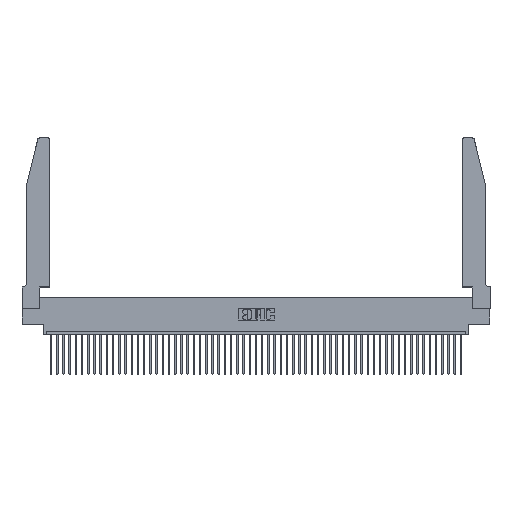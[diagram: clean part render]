
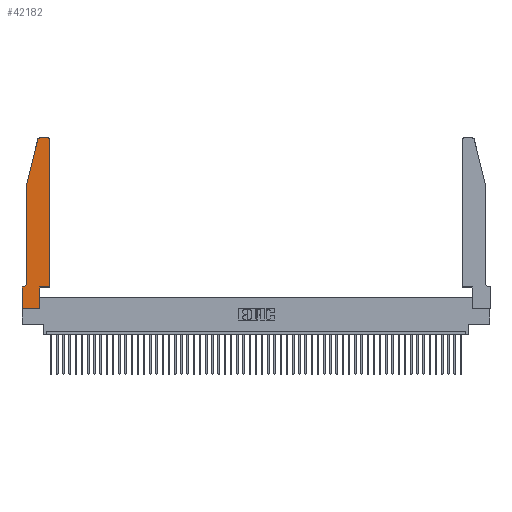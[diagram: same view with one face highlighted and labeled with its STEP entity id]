
A CAD part, top view. The second image highlights one B-rep face of the part: STEP entity #42182.
In plain terms, the highlighted planar face has unit normal (0, 0, 1).
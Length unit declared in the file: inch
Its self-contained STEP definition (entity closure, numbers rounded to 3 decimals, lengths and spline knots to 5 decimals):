
#329 = CARTESIAN_POINT ( 'NONE',  ( 0.0755, 2., 0.37 ) ) ;
#346 = CIRCLE ( 'NONE', #16321, 0.03 ) ;
#608 = CARTESIAN_POINT ( 'NONE',  ( 0.4205, 2.75, 0.37 ) ) ;
#886 = VERTEX_POINT ( 'NONE', #20206 ) ;
#1079 = VERTEX_POINT ( 'NONE', #32939 ) ;
#1158 = CARTESIAN_POINT ( 'NONE',  ( 0.0755, 2., 0.37 ) ) ;
#1181 = CARTESIAN_POINT ( 'NONE',  ( 0.0055, 0.42, 0.37 ) ) ;
#2840 = CARTESIAN_POINT ( 'NONE',  ( 0., 0., 0.37 ) ) ;
#4783 = DIRECTION ( 'NONE',  ( -1., 0., 0. ) ) ;
#4904 = DIRECTION ( 'NONE',  ( 0., 0., 1. ) ) ;
#5257 = DIRECTION ( 'NONE',  ( 0., 0., -1. ) ) ;
#5726 = AXIS2_PLACEMENT_3D ( 'NONE', #1181, #5257, #4783 ) ;
#6434 = EDGE_CURVE ( 'NONE', #24270, #14712, #34978, .T. ) ;
#6566 = VECTOR ( 'NONE', #10923, 39.37008 ) ;
#6941 = CARTESIAN_POINT ( 'NONE',  ( 0.4505, 2.72, 0.37 ) ) ;
#7412 = EDGE_CURVE ( 'NONE', #33512, #45178, #346, .T. ) ;
#9085 = EDGE_CURVE ( 'NONE', #45178, #26135, #44754, .T. ) ;
#9306 = DIRECTION ( 'NONE',  ( -0.239, -0.971, 0. ) ) ;
#10079 = VECTOR ( 'NONE', #38637, 39.37008 ) ;
#10217 = ORIENTED_EDGE ( 'NONE', *, *, #29654, .T. ) ;
#10428 = CARTESIAN_POINT ( 'NONE',  ( 0.4505, 0.35, 0.37 ) ) ;
#10923 = DIRECTION ( 'NONE',  ( 1., 0., 0. ) ) ;
#11467 = DIRECTION ( 'NONE',  ( -1., 0., 0. ) ) ;
#11784 = ORIENTED_EDGE ( 'NONE', *, *, #13520, .T. ) ;
#12671 = CARTESIAN_POINT ( 'NONE',  ( 0.4205, 2.72, 0.37 ) ) ;
#13118 = ORIENTED_EDGE ( 'NONE', *, *, #25463, .T. ) ;
#13520 = EDGE_CURVE ( 'NONE', #48014, #1079, #25300, .T. ) ;
#13732 = ORIENTED_EDGE ( 'NONE', *, *, #50734, .T. ) ;
#13785 = ORIENTED_EDGE ( 'NONE', *, *, #41530, .T. ) ;
#13830 = CARTESIAN_POINT ( 'NONE',  ( 0., 0.35, 0.37 ) ) ;
#14712 = VERTEX_POINT ( 'NONE', #1158 ) ;
#16321 = AXIS2_PLACEMENT_3D ( 'NONE', #12671, #19629, #17444 ) ;
#16602 = CARTESIAN_POINT ( 'NONE',  ( 0.25487, 2.72718, 0.37 ) ) ;
#17444 = DIRECTION ( 'NONE',  ( 1., 0., 0. ) ) ;
#17560 = ORIENTED_EDGE ( 'NONE', *, *, #6434, .T. ) ;
#18526 = ORIENTED_EDGE ( 'NONE', *, *, #9085, .T. ) ;
#19629 = DIRECTION ( 'NONE',  ( 0., 0., 1. ) ) ;
#20206 = CARTESIAN_POINT ( 'NONE',  ( 0.2865, 0., 0.37 ) ) ;
#20846 = LINE ( 'NONE', #45783, #51083 ) ;
#21746 = DIRECTION ( 'NONE',  ( 1., 0., 0. ) ) ;
#21899 = VERTEX_POINT ( 'NONE', #38941 ) ;
#22850 = CARTESIAN_POINT ( 'NONE',  ( 0.2605, 2.75, 0.37 ) ) ;
#23298 = EDGE_CURVE ( 'NONE', #42339, #886, #20846, .T. ) ;
#24270 = VERTEX_POINT ( 'NONE', #16602 ) ;
#24715 = VECTOR ( 'NONE', #26577, 39.37008 ) ;
#24880 = CARTESIAN_POINT ( 'NONE',  ( 0.284, 2.72, 0.37 ) ) ;
#25300 = LINE ( 'NONE', #34911, #6566 ) ;
#25463 = EDGE_CURVE ( 'NONE', #1079, #33512, #35424, .T. ) ;
#26110 = EDGE_CURVE ( 'NONE', #26135, #24270, #37158, .T. ) ;
#26112 = DIRECTION ( 'NONE',  ( 0., 0., 1. ) ) ;
#26135 = VERTEX_POINT ( 'NONE', #30339 ) ;
#26250 = LINE ( 'NONE', #329, #51472 ) ;
#26326 = CARTESIAN_POINT ( 'NONE',  ( 0.2865, 0.35, 0.37 ) ) ;
#26564 = VECTOR ( 'NONE', #38978, 39.37008 ) ;
#26577 = DIRECTION ( 'NONE',  ( 0., 1., 0. ) ) ;
#27135 = ORIENTED_EDGE ( 'NONE', *, *, #26110, .T. ) ;
#27456 = CARTESIAN_POINT ( 'NONE',  ( 0.0755, 2., 0.37 ) ) ;
#27586 = CARTESIAN_POINT ( 'NONE',  ( 0.0755, 0.35, 0.37 ) ) ;
#29398 = CARTESIAN_POINT ( 'NONE',  ( 0.2865, 0.35, 0.37 ) ) ;
#29490 = LINE ( 'NONE', #26326, #10079 ) ;
#29654 = EDGE_CURVE ( 'NONE', #32165, #21899, #34146, .T. ) ;
#29679 = CARTESIAN_POINT ( 'NONE',  ( 0., 0., 0.37 ) ) ;
#29783 = FACE_OUTER_BOUND ( 'NONE', #38321, .T. ) ;
#30339 = CARTESIAN_POINT ( 'NONE',  ( 0.284, 2.75, 0.37 ) ) ;
#30767 = VECTOR ( 'NONE', #41751, 39.37008 ) ;
#32165 = VERTEX_POINT ( 'NONE', #45213 ) ;
#32939 = CARTESIAN_POINT ( 'NONE',  ( 0.4505, 0.35, 0.37 ) ) ;
#33512 = VERTEX_POINT ( 'NONE', #6941 ) ;
#34146 = LINE ( 'NONE', #27586, #50504 ) ;
#34911 = CARTESIAN_POINT ( 'NONE',  ( 0.4505, 0.35, 0.37 ) ) ;
#34978 = LINE ( 'NONE', #27456, #48210 ) ;
#35424 = LINE ( 'NONE', #10428, #24715 ) ;
#35716 = ORIENTED_EDGE ( 'NONE', *, *, #43220, .T. ) ;
#36349 = LINE ( 'NONE', #29679, #30767 ) ;
#37158 = CIRCLE ( 'NONE', #46968, 0.03 ) ;
#37225 = ORIENTED_EDGE ( 'NONE', *, *, #49859, .T. ) ;
#38321 = EDGE_LOOP ( 'NONE', ( #18526, #27135, #17560, #13732, #35716, #10217, #13785, #46394, #37225, #11784, #13118, #49181 ) ) ;
#38637 = DIRECTION ( 'NONE',  ( 0., 1., 0. ) ) ;
#38941 = CARTESIAN_POINT ( 'NONE',  ( 0., 0.35, 0.37 ) ) ;
#38967 = VERTEX_POINT ( 'NONE', #43583 ) ;
#38978 = DIRECTION ( 'NONE',  ( -1., 0., 0. ) ) ;
#39126 = CIRCLE ( 'NONE', #5726, 0.07 ) ;
#40302 = DIRECTION ( 'NONE',  ( 0., -1., 0. ) ) ;
#41334 = DIRECTION ( 'NONE',  ( 1., 0., 0. ) ) ;
#41530 = EDGE_CURVE ( 'NONE', #21899, #42339, #36349, .T. ) ;
#41751 = DIRECTION ( 'NONE',  ( 0., -1., 0. ) ) ;
#42045 = PLANE ( 'NONE',  #48416 ) ;
#42182 = ADVANCED_FACE ( 'NONE', ( #29783 ), #42045, .T. ) ;
#42339 = VERTEX_POINT ( 'NONE', #2840 ) ;
#43220 = EDGE_CURVE ( 'NONE', #38967, #32165, #39126, .T. ) ;
#43583 = CARTESIAN_POINT ( 'NONE',  ( 0.0755, 0.42, 0.37 ) ) ;
#44754 = LINE ( 'NONE', #22850, #26564 ) ;
#45178 = VERTEX_POINT ( 'NONE', #608 ) ;
#45213 = CARTESIAN_POINT ( 'NONE',  ( 0.0055, 0.35, 0.37 ) ) ;
#45783 = CARTESIAN_POINT ( 'NONE',  ( 0., 0., 0.37 ) ) ;
#46394 = ORIENTED_EDGE ( 'NONE', *, *, #23298, .T. ) ;
#46968 = AXIS2_PLACEMENT_3D ( 'NONE', #24880, #4904, #48439 ) ;
#48014 = VERTEX_POINT ( 'NONE', #29398 ) ;
#48210 = VECTOR ( 'NONE', #9306, 39.37008 ) ;
#48416 = AXIS2_PLACEMENT_3D ( 'NONE', #13830, #26112, #41334 ) ;
#48439 = DIRECTION ( 'NONE',  ( 1., 0., 0. ) ) ;
#49181 = ORIENTED_EDGE ( 'NONE', *, *, #7412, .T. ) ;
#49859 = EDGE_CURVE ( 'NONE', #886, #48014, #29490, .T. ) ;
#50504 = VECTOR ( 'NONE', #11467, 39.37008 ) ;
#50734 = EDGE_CURVE ( 'NONE', #14712, #38967, #26250, .T. ) ;
#51083 = VECTOR ( 'NONE', #21746, 39.37008 ) ;
#51472 = VECTOR ( 'NONE', #40302, 39.37008 ) ;
